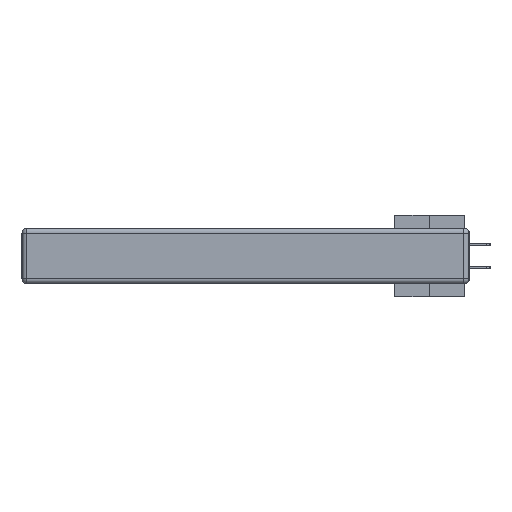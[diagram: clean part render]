
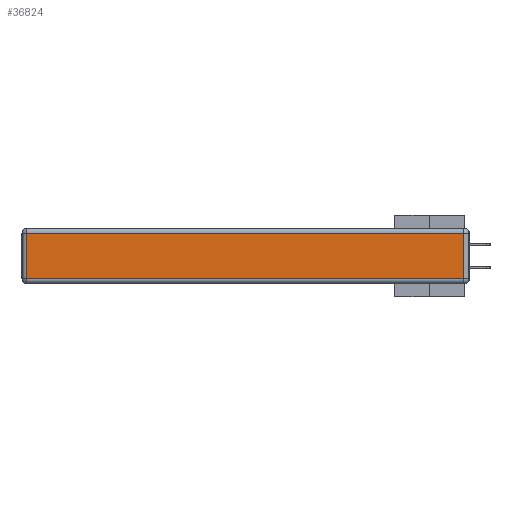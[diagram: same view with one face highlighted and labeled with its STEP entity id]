
A CAD part, left-side view. The second image highlights one B-rep face of the part: STEP entity #36824.
In plain terms, the highlighted planar face has unit normal (-1, 0, 0).
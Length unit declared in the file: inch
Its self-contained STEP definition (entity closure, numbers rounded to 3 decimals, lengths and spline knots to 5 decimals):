
#1164 = LINE ( 'NONE', #38610, #1788 ) ;
#1537 = VECTOR ( 'NONE', #2438, 39.37008 ) ;
#1788 = VECTOR ( 'NONE', #38931, 39.37008 ) ;
#2418 = ORIENTED_EDGE ( 'NONE', *, *, #39184, .T. ) ;
#2438 = DIRECTION ( 'NONE',  ( 0., 1., 0. ) ) ;
#4821 = DIRECTION ( 'NONE',  ( 0., 0., -1. ) ) ;
#8038 = CARTESIAN_POINT ( 'NONE',  ( 0., 0.03, -0.313 ) ) ;
#8812 = EDGE_CURVE ( 'NONE', #21488, #11177, #14016, .T. ) ;
#9910 = CARTESIAN_POINT ( 'NONE',  ( 0., 0.03, -0.03 ) ) ;
#11177 = VERTEX_POINT ( 'NONE', #9910 ) ;
#11606 = ORIENTED_EDGE ( 'NONE', *, *, #46787, .T. ) ;
#11624 = LINE ( 'NONE', #21985, #1537 ) ;
#11682 = CARTESIAN_POINT ( 'NONE',  ( 0., 0.03, -0.343 ) ) ;
#14016 = LINE ( 'NONE', #11682, #27663 ) ;
#19092 = VECTOR ( 'NONE', #4821, 39.37008 ) ;
#19377 = VERTEX_POINT ( 'NONE', #24177 ) ;
#20554 = ORIENTED_EDGE ( 'NONE', *, *, #28521, .T. ) ;
#21488 = VERTEX_POINT ( 'NONE', #8038 ) ;
#21879 = PLANE ( 'NONE',  #36742 ) ;
#21985 = CARTESIAN_POINT ( 'NONE',  ( 0., 2.75, -0.03 ) ) ;
#24177 = CARTESIAN_POINT ( 'NONE',  ( 0., 2.72, -0.03 ) ) ;
#27129 = VERTEX_POINT ( 'NONE', #33434 ) ;
#27411 = FACE_OUTER_BOUND ( 'NONE', #37027, .T. ) ;
#27663 = VECTOR ( 'NONE', #30881, 39.37008 ) ;
#28521 = EDGE_CURVE ( 'NONE', #19377, #27129, #45766, .T. ) ;
#29485 = DIRECTION ( 'NONE',  ( -1., 0., 0. ) ) ;
#30449 = ORIENTED_EDGE ( 'NONE', *, *, #8812, .T. ) ;
#30881 = DIRECTION ( 'NONE',  ( 0., 0., 1. ) ) ;
#33310 = DIRECTION ( 'NONE',  ( 0., 0., 1. ) ) ;
#33434 = CARTESIAN_POINT ( 'NONE',  ( 0., 2.72, -0.313 ) ) ;
#36742 = AXIS2_PLACEMENT_3D ( 'NONE', #40930, #29485, #33310 ) ;
#36824 = ADVANCED_FACE ( 'NONE', ( #27411 ), #21879, .T. ) ;
#37027 = EDGE_LOOP ( 'NONE', ( #2418, #30449, #11606, #20554 ) ) ;
#38610 = CARTESIAN_POINT ( 'NONE',  ( 0., 0., -0.313 ) ) ;
#38931 = DIRECTION ( 'NONE',  ( 0., -1., 0. ) ) ;
#39184 = EDGE_CURVE ( 'NONE', #27129, #21488, #1164, .T. ) ;
#40930 = CARTESIAN_POINT ( 'NONE',  ( 0., 0., -0.343 ) ) ;
#45766 = LINE ( 'NONE', #46269, #19092 ) ;
#46269 = CARTESIAN_POINT ( 'NONE',  ( 0., 2.72, -0.343 ) ) ;
#46787 = EDGE_CURVE ( 'NONE', #11177, #19377, #11624, .T. ) ;
